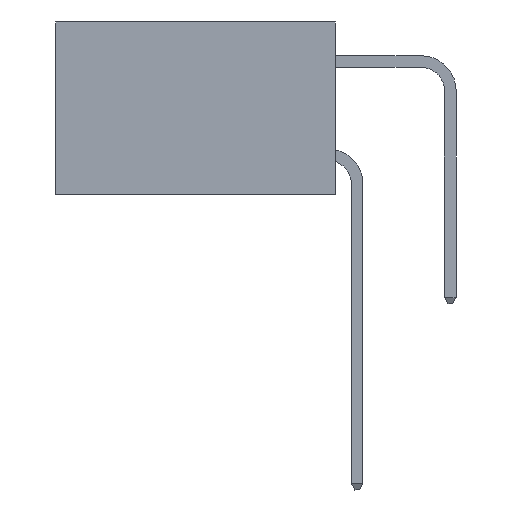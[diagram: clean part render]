
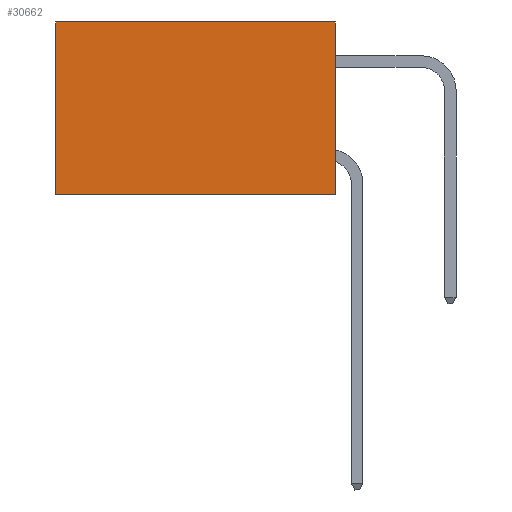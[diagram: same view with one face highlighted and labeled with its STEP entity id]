
A CAD part, left-side view. The second image highlights one B-rep face of the part: STEP entity #30662.
In plain terms, the highlighted planar face has unit normal (-1, 0, 0).
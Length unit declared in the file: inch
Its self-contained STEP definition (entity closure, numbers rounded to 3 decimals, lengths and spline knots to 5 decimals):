
#703 = VECTOR ( 'NONE', #11213, 39.37008 ) ;
#1680 = EDGE_LOOP ( 'NONE', ( #5718, #21023, #23718, #8354 ) ) ;
#2582 = DIRECTION ( 'NONE',  ( 1., 0., 0. ) ) ;
#5718 = ORIENTED_EDGE ( 'NONE', *, *, #34023, .T. ) ;
#6784 = LINE ( 'NONE', #20773, #21107 ) ;
#6786 = VERTEX_POINT ( 'NONE', #14397 ) ;
#8354 = ORIENTED_EDGE ( 'NONE', *, *, #24655, .T. ) ;
#8543 = VERTEX_POINT ( 'NONE', #35509 ) ;
#9058 = VERTEX_POINT ( 'NONE', #32473 ) ;
#9260 = LINE ( 'NONE', #25498, #703 ) ;
#10903 = VERTEX_POINT ( 'NONE', #34963 ) ;
#11213 = DIRECTION ( 'NONE',  ( 0., 1., 0. ) ) ;
#11949 = LINE ( 'NONE', #21747, #18705 ) ;
#12379 = VECTOR ( 'NONE', #19878, 39.37008 ) ;
#12977 = AXIS2_PLACEMENT_3D ( 'NONE', #19768, #2582, #22625 ) ;
#14055 = FACE_OUTER_BOUND ( 'NONE', #1680, .T. ) ;
#14397 = CARTESIAN_POINT ( 'NONE',  ( 0.2875, 0., -0.37 ) ) ;
#16188 = DIRECTION ( 'NONE',  ( 0., 1., 0. ) ) ;
#18705 = VECTOR ( 'NONE', #16188, 39.37008 ) ;
#19768 = CARTESIAN_POINT ( 'NONE',  ( 0.2875, 0., 0. ) ) ;
#19878 = DIRECTION ( 'NONE',  ( 0., 0., -1. ) ) ;
#19999 = CARTESIAN_POINT ( 'NONE',  ( 0.2875, 0.6, 0. ) ) ;
#20773 = CARTESIAN_POINT ( 'NONE',  ( 0.2875, 0., 0. ) ) ;
#21023 = ORIENTED_EDGE ( 'NONE', *, *, #21760, .F. ) ;
#21107 = VECTOR ( 'NONE', #23641, 39.37008 ) ;
#21747 = CARTESIAN_POINT ( 'NONE',  ( 0.2875, 0., -0.37 ) ) ;
#21760 = EDGE_CURVE ( 'NONE', #6786, #10903, #11949, .T. ) ;
#22625 = DIRECTION ( 'NONE',  ( 0., 0., -1. ) ) ;
#23641 = DIRECTION ( 'NONE',  ( 0., 0., -1. ) ) ;
#23718 = ORIENTED_EDGE ( 'NONE', *, *, #27819, .F. ) ;
#24655 = EDGE_CURVE ( 'NONE', #8543, #9058, #9260, .T. ) ;
#25498 = CARTESIAN_POINT ( 'NONE',  ( 0.2875, 0., 0. ) ) ;
#27631 = LINE ( 'NONE', #19999, #12379 ) ;
#27819 = EDGE_CURVE ( 'NONE', #8543, #6786, #6784, .T. ) ;
#28288 = PLANE ( 'NONE',  #12977 ) ;
#30662 = ADVANCED_FACE ( 'NONE', ( #14055 ), #28288, .F. ) ;
#32473 = CARTESIAN_POINT ( 'NONE',  ( 0.2875, 0.6, 0. ) ) ;
#34023 = EDGE_CURVE ( 'NONE', #9058, #10903, #27631, .T. ) ;
#34963 = CARTESIAN_POINT ( 'NONE',  ( 0.2875, 0.6, -0.37 ) ) ;
#35509 = CARTESIAN_POINT ( 'NONE',  ( 0.2875, 0., 0. ) ) ;
